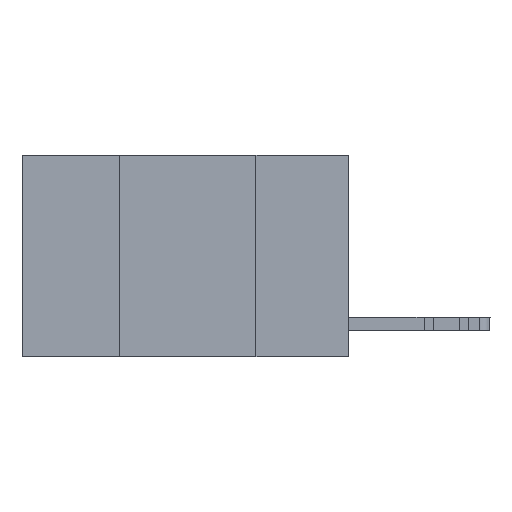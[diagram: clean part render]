
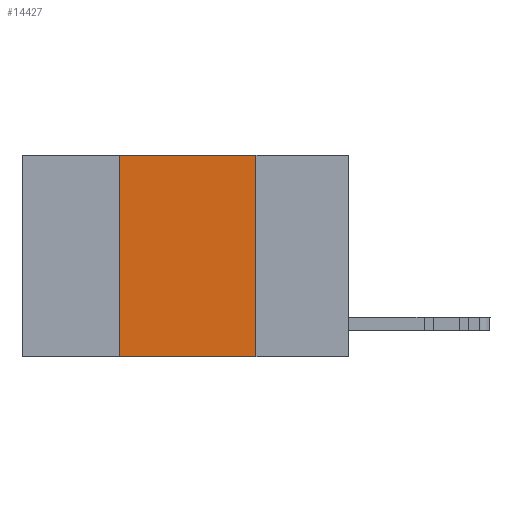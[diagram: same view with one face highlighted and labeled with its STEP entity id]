
A CAD part, left-side view. The second image highlights one B-rep face of the part: STEP entity #14427.
In plain terms, the highlighted planar face has unit normal (-1, 0, 0).
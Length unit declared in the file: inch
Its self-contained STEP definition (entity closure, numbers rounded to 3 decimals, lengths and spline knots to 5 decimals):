
#548 = ORIENTED_EDGE ( 'NONE', *, *, #27481, .F. ) ;
#1713 = ORIENTED_EDGE ( 'NONE', *, *, #22498, .F. ) ;
#1797 = EDGE_CURVE ( 'NONE', #11249, #20855, #5560, .T. ) ;
#2211 = ORIENTED_EDGE ( 'NONE', *, *, #1797, .F. ) ;
#2267 = VERTEX_POINT ( 'NONE', #25157 ) ;
#4567 = CARTESIAN_POINT ( 'NONE',  ( 0., 0.6, 0. ) ) ;
#4808 = VECTOR ( 'NONE', #5471, 39.37008 ) ;
#5471 = DIRECTION ( 'NONE',  ( 0., 0., 1. ) ) ;
#5560 = LINE ( 'NONE', #27831, #17431 ) ;
#5980 = CARTESIAN_POINT ( 'NONE',  ( 0., 0.17, -0.37 ) ) ;
#6605 = CARTESIAN_POINT ( 'NONE',  ( 0., 0.6, -0.37 ) ) ;
#6740 = LINE ( 'NONE', #25855, #12749 ) ;
#9929 = CARTESIAN_POINT ( 'NONE',  ( 0., 0.42, 0. ) ) ;
#10850 = LINE ( 'NONE', #9929, #4808 ) ;
#11128 = VERTEX_POINT ( 'NONE', #16374 ) ;
#11249 = VERTEX_POINT ( 'NONE', #18842 ) ;
#11374 = DIRECTION ( 'NONE',  ( 1., 0., 0. ) ) ;
#12162 = ORIENTED_EDGE ( 'NONE', *, *, #26053, .T. ) ;
#12749 = VECTOR ( 'NONE', #21580, 39.37008 ) ;
#14404 = VECTOR ( 'NONE', #24189, 39.37008 ) ;
#14427 = ADVANCED_FACE ( 'NONE', ( #21896 ), #24491, .F. ) ;
#16374 = CARTESIAN_POINT ( 'NONE',  ( 0., 0.42, 0. ) ) ;
#16991 = DIRECTION ( 'NONE',  ( 0., 0., -1. ) ) ;
#17431 = VECTOR ( 'NONE', #16991, 39.37008 ) ;
#18842 = CARTESIAN_POINT ( 'NONE',  ( 0., 0.17, 0. ) ) ;
#20197 = LINE ( 'NONE', #6605, #14404 ) ;
#20812 = EDGE_LOOP ( 'NONE', ( #2211, #1713, #548, #12162 ) ) ;
#20855 = VERTEX_POINT ( 'NONE', #5980 ) ;
#21580 = DIRECTION ( 'NONE',  ( 0., -1., 0. ) ) ;
#21863 = AXIS2_PLACEMENT_3D ( 'NONE', #4567, #11374, #26693 ) ;
#21896 = FACE_OUTER_BOUND ( 'NONE', #20812, .T. ) ;
#22498 = EDGE_CURVE ( 'NONE', #11128, #11249, #6740, .T. ) ;
#24189 = DIRECTION ( 'NONE',  ( 0., -1., 0. ) ) ;
#24491 = PLANE ( 'NONE',  #21863 ) ;
#25157 = CARTESIAN_POINT ( 'NONE',  ( 0., 0.42, -0.37 ) ) ;
#25855 = CARTESIAN_POINT ( 'NONE',  ( 0., 0.6, 0. ) ) ;
#26053 = EDGE_CURVE ( 'NONE', #2267, #20855, #20197, .T. ) ;
#26693 = DIRECTION ( 'NONE',  ( 0., 0., -1. ) ) ;
#27481 = EDGE_CURVE ( 'NONE', #2267, #11128, #10850, .T. ) ;
#27831 = CARTESIAN_POINT ( 'NONE',  ( 0., 0.17, 0. ) ) ;
